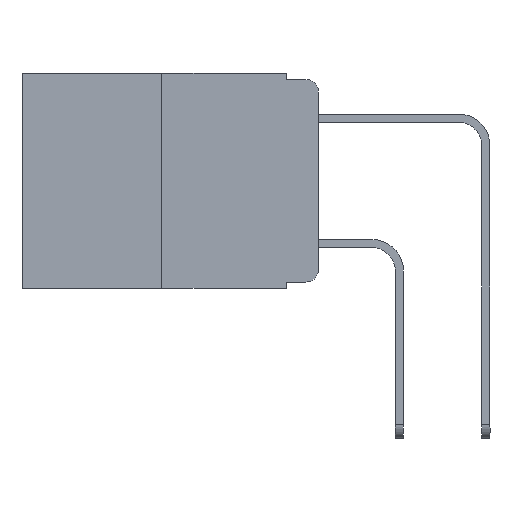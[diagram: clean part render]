
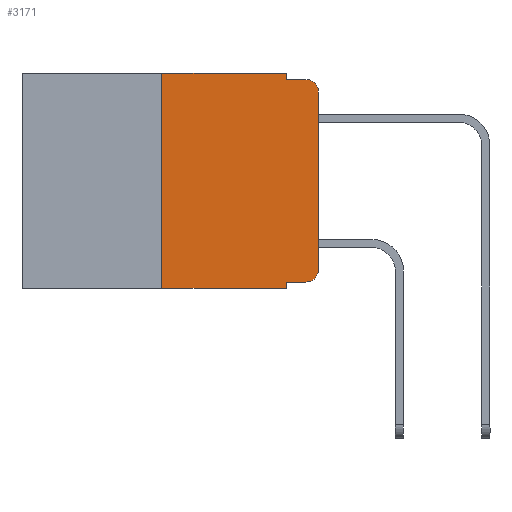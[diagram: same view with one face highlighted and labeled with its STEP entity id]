
A CAD part, left-side view. The second image highlights one B-rep face of the part: STEP entity #3171.
In plain terms, the highlighted planar face has unit normal (-1, 0, 0).
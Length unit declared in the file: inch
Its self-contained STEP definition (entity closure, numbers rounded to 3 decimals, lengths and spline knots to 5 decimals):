
#104 = EDGE_CURVE ( 'NONE', #15858, #5092, #9654, .T. ) ;
#206 = EDGE_CURVE ( 'NONE', #7686, #3578, #10496, .T. ) ;
#606 = EDGE_CURVE ( 'NONE', #3578, #4813, #6180, .T. ) ;
#623 = CARTESIAN_POINT ( 'NONE',  ( 0., 0.051, 0. ) ) ;
#722 = LINE ( 'NONE', #7505, #9616 ) ;
#736 = VECTOR ( 'NONE', #5764, 39.37008 ) ;
#885 = DIRECTION ( 'NONE',  ( -1., 0., 0. ) ) ;
#896 = CARTESIAN_POINT ( 'NONE',  ( 0., 0.25, -0.343 ) ) ;
#1036 = CARTESIAN_POINT ( 'NONE',  ( 0., 0., 0. ) ) ;
#1138 = EDGE_CURVE ( 'NONE', #15126, #12684, #12533, .T. ) ;
#1316 = DIRECTION ( 'NONE',  ( 0., 0., -1. ) ) ;
#1788 = VERTEX_POINT ( 'NONE', #13599 ) ;
#2248 = EDGE_CURVE ( 'NONE', #15858, #7686, #722, .T. ) ;
#2275 = DIRECTION ( 'NONE',  ( 0., -1., 0. ) ) ;
#2309 = VERTEX_POINT ( 'NONE', #896 ) ;
#2352 = CARTESIAN_POINT ( 'NONE',  ( 0., 0.02, -0.03 ) ) ;
#2455 = DIRECTION ( 'NONE',  ( 0., -1., 0. ) ) ;
#3157 = DIRECTION ( 'NONE',  ( 0., -1., 0. ) ) ;
#3171 = ADVANCED_FACE ( 'NONE', ( #9935 ), #16580, .F. ) ;
#3578 = VERTEX_POINT ( 'NONE', #4760 ) ;
#3721 = DIRECTION ( 'NONE',  ( 0., 0., -1. ) ) ;
#3744 = ORIENTED_EDGE ( 'NONE', *, *, #15066, .T. ) ;
#3746 = ORIENTED_EDGE ( 'NONE', *, *, #104, .F. ) ;
#4111 = EDGE_CURVE ( 'NONE', #2309, #1788, #10328, .T. ) ;
#4281 = VECTOR ( 'NONE', #2455, 39.37008 ) ;
#4470 = CARTESIAN_POINT ( 'NONE',  ( 0., 0.051, -0.333 ) ) ;
#4760 = CARTESIAN_POINT ( 'NONE',  ( 0., 0., -0.313 ) ) ;
#4813 = VERTEX_POINT ( 'NONE', #12843 ) ;
#5092 = VERTEX_POINT ( 'NONE', #12319 ) ;
#5178 = CARTESIAN_POINT ( 'NONE',  ( 0., 0.051, -0.01 ) ) ;
#5575 = VECTOR ( 'NONE', #10052, 39.37008 ) ;
#5764 = DIRECTION ( 'NONE',  ( 0., 0., -1. ) ) ;
#5979 = CARTESIAN_POINT ( 'NONE',  ( 0., 0.473, -0.343 ) ) ;
#6180 = LINE ( 'NONE', #1036, #5575 ) ;
#6393 = CARTESIAN_POINT ( 'NONE',  ( 0., 0.473, 0. ) ) ;
#7145 = ORIENTED_EDGE ( 'NONE', *, *, #606, .T. ) ;
#7342 = VECTOR ( 'NONE', #3157, 39.37008 ) ;
#7505 = CARTESIAN_POINT ( 'NONE',  ( 0., 0.051, -0.333 ) ) ;
#7571 = DIRECTION ( 'NONE',  ( 0., 0., 1. ) ) ;
#7686 = VERTEX_POINT ( 'NONE', #7889 ) ;
#7889 = CARTESIAN_POINT ( 'NONE',  ( 0., 0.02, -0.333 ) ) ;
#8408 = EDGE_CURVE ( 'NONE', #2309, #5092, #13633, .T. ) ;
#8598 = ORIENTED_EDGE ( 'NONE', *, *, #9990, .F. ) ;
#8638 = ORIENTED_EDGE ( 'NONE', *, *, #8408, .T. ) ;
#8778 = CARTESIAN_POINT ( 'NONE',  ( 0., 0.02, -0.313 ) ) ;
#8858 = DIRECTION ( 'NONE',  ( 0., 0., -1. ) ) ;
#8937 = VERTEX_POINT ( 'NONE', #623 ) ;
#8945 = CARTESIAN_POINT ( 'NONE',  ( 0., 0.051, 0. ) ) ;
#9446 = CARTESIAN_POINT ( 'NONE',  ( 0., 0.051, 0. ) ) ;
#9616 = VECTOR ( 'NONE', #2275, 39.37008 ) ;
#9654 = LINE ( 'NONE', #8945, #14894 ) ;
#9715 = AXIS2_PLACEMENT_3D ( 'NONE', #13824, #11491, #13990 ) ;
#9764 = ORIENTED_EDGE ( 'NONE', *, *, #11034, .F. ) ;
#9935 = FACE_OUTER_BOUND ( 'NONE', #11604, .T. ) ;
#9990 = EDGE_CURVE ( 'NONE', #1788, #8937, #10093, .T. ) ;
#10052 = DIRECTION ( 'NONE',  ( 0., 0., 1. ) ) ;
#10093 = LINE ( 'NONE', #6393, #4281 ) ;
#10328 = LINE ( 'NONE', #15589, #14419 ) ;
#10483 = AXIS2_PLACEMENT_3D ( 'NONE', #8778, #885, #3721 ) ;
#10496 = CIRCLE ( 'NONE', #10483, 0.02 ) ;
#11034 = EDGE_CURVE ( 'NONE', #8937, #15126, #14615, .T. ) ;
#11244 = CARTESIAN_POINT ( 'NONE',  ( 0., 0.051, -0.01 ) ) ;
#11491 = DIRECTION ( 'NONE',  ( 1., 0., 0. ) ) ;
#11604 = EDGE_LOOP ( 'NONE', ( #7145, #3744, #12101, #9764, #8598, #14077, #8638, #3746, #16380, #12140 ) ) ;
#11607 = CARTESIAN_POINT ( 'NONE',  ( 0., 0.02, -0.01 ) ) ;
#12101 = ORIENTED_EDGE ( 'NONE', *, *, #1138, .F. ) ;
#12140 = ORIENTED_EDGE ( 'NONE', *, *, #206, .T. ) ;
#12319 = CARTESIAN_POINT ( 'NONE',  ( 0., 0.051, -0.343 ) ) ;
#12533 = LINE ( 'NONE', #11244, #14945 ) ;
#12684 = VERTEX_POINT ( 'NONE', #11607 ) ;
#12843 = CARTESIAN_POINT ( 'NONE',  ( 0., 0., -0.03 ) ) ;
#13599 = CARTESIAN_POINT ( 'NONE',  ( 0., 0.25, 0. ) ) ;
#13633 = LINE ( 'NONE', #5979, #7342 ) ;
#13824 = CARTESIAN_POINT ( 'NONE',  ( 0., 0.473, 0. ) ) ;
#13990 = DIRECTION ( 'NONE',  ( 0., 0., -1. ) ) ;
#14077 = ORIENTED_EDGE ( 'NONE', *, *, #4111, .F. ) ;
#14419 = VECTOR ( 'NONE', #7571, 39.37008 ) ;
#14615 = LINE ( 'NONE', #9446, #736 ) ;
#14894 = VECTOR ( 'NONE', #8858, 39.37008 ) ;
#14945 = VECTOR ( 'NONE', #16512, 39.37008 ) ;
#15066 = EDGE_CURVE ( 'NONE', #4813, #12684, #16477, .T. ) ;
#15126 = VERTEX_POINT ( 'NONE', #5178 ) ;
#15423 = DIRECTION ( 'NONE',  ( -1., 0., 0. ) ) ;
#15589 = CARTESIAN_POINT ( 'NONE',  ( 0., 0.25, 0. ) ) ;
#15651 = AXIS2_PLACEMENT_3D ( 'NONE', #2352, #15423, #1316 ) ;
#15858 = VERTEX_POINT ( 'NONE', #4470 ) ;
#16380 = ORIENTED_EDGE ( 'NONE', *, *, #2248, .T. ) ;
#16477 = CIRCLE ( 'NONE', #15651, 0.02 ) ;
#16512 = DIRECTION ( 'NONE',  ( 0., -1., 0. ) ) ;
#16580 = PLANE ( 'NONE',  #9715 ) ;
